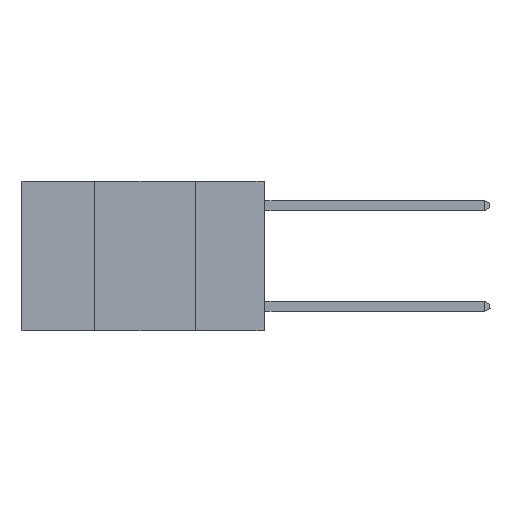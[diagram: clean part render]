
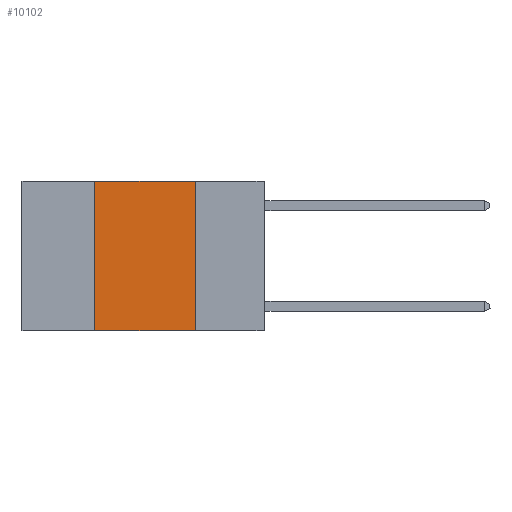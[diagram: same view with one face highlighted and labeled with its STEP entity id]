
A CAD part, left-side view. The second image highlights one B-rep face of the part: STEP entity #10102.
In plain terms, the highlighted planar face has unit normal (-1, 0, 0).
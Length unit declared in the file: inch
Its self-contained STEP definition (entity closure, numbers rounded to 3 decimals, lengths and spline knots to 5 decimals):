
#408 = VECTOR ( 'NONE', #20294, 39.37008 ) ;
#576 = ORIENTED_EDGE ( 'NONE', *, *, #16617, .F. ) ;
#1001 = ORIENTED_EDGE ( 'NONE', *, *, #7773, .T. ) ;
#1592 = CARTESIAN_POINT ( 'NONE',  ( 0., 0.17, -0.37 ) ) ;
#1856 = ORIENTED_EDGE ( 'NONE', *, *, #7133, .F. ) ;
#2505 = VECTOR ( 'NONE', #2964, 39.37008 ) ;
#2964 = DIRECTION ( 'NONE',  ( 0., 0., -1. ) ) ;
#3948 = LINE ( 'NONE', #12137, #408 ) ;
#4323 = CARTESIAN_POINT ( 'NONE',  ( 0., 0.42, 0. ) ) ;
#4561 = VERTEX_POINT ( 'NONE', #9157 ) ;
#6222 = LINE ( 'NONE', #11442, #25142 ) ;
#7003 = LINE ( 'NONE', #17164, #2505 ) ;
#7133 = EDGE_CURVE ( 'NONE', #4561, #12014, #7003, .T. ) ;
#7671 = CARTESIAN_POINT ( 'NONE',  ( 0., 0.6, 0. ) ) ;
#7773 = EDGE_CURVE ( 'NONE', #21719, #12014, #3948, .T. ) ;
#8984 = LINE ( 'NONE', #25309, #25013 ) ;
#9157 = CARTESIAN_POINT ( 'NONE',  ( 0., 0.17, 0. ) ) ;
#9455 = EDGE_LOOP ( 'NONE', ( #1856, #576, #11302, #1001 ) ) ;
#10102 = ADVANCED_FACE ( 'NONE', ( #15829 ), #13702, .F. ) ;
#11302 = ORIENTED_EDGE ( 'NONE', *, *, #22263, .F. ) ;
#11442 = CARTESIAN_POINT ( 'NONE',  ( 0., 0.42, 0. ) ) ;
#12014 = VERTEX_POINT ( 'NONE', #1592 ) ;
#12137 = CARTESIAN_POINT ( 'NONE',  ( 0., 0.6, -0.37 ) ) ;
#13702 = PLANE ( 'NONE',  #17891 ) ;
#15829 = FACE_OUTER_BOUND ( 'NONE', #9455, .T. ) ;
#16617 = EDGE_CURVE ( 'NONE', #18456, #4561, #8984, .T. ) ;
#17004 = DIRECTION ( 'NONE',  ( 0., -1., 0. ) ) ;
#17164 = CARTESIAN_POINT ( 'NONE',  ( 0., 0.17, 0. ) ) ;
#17891 = AXIS2_PLACEMENT_3D ( 'NONE', #7671, #23998, #19574 ) ;
#18456 = VERTEX_POINT ( 'NONE', #4323 ) ;
#19464 = DIRECTION ( 'NONE',  ( 0., 0., 1. ) ) ;
#19574 = DIRECTION ( 'NONE',  ( 0., 0., -1. ) ) ;
#20294 = DIRECTION ( 'NONE',  ( 0., -1., 0. ) ) ;
#20581 = CARTESIAN_POINT ( 'NONE',  ( 0., 0.42, -0.37 ) ) ;
#21719 = VERTEX_POINT ( 'NONE', #20581 ) ;
#22263 = EDGE_CURVE ( 'NONE', #21719, #18456, #6222, .T. ) ;
#23998 = DIRECTION ( 'NONE',  ( 1., 0., 0. ) ) ;
#25013 = VECTOR ( 'NONE', #17004, 39.37008 ) ;
#25142 = VECTOR ( 'NONE', #19464, 39.37008 ) ;
#25309 = CARTESIAN_POINT ( 'NONE',  ( 0., 0.6, 0. ) ) ;
